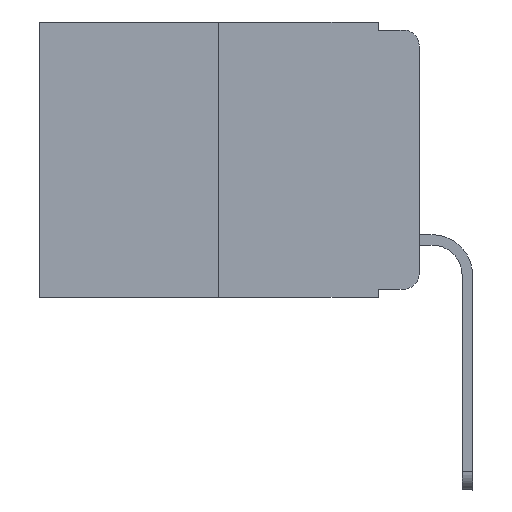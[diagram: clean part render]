
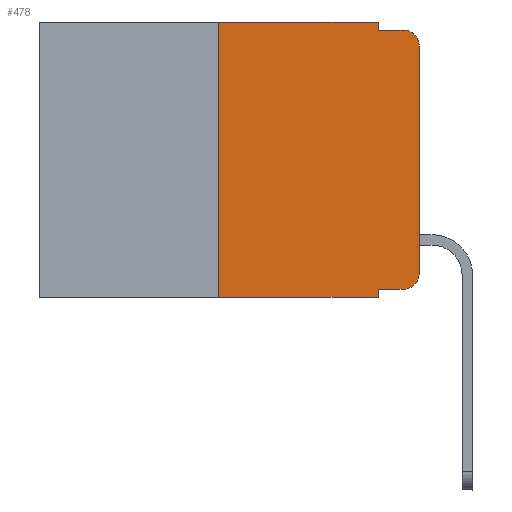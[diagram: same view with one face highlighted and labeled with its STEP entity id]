
A CAD part, left-side view. The second image highlights one B-rep face of the part: STEP entity #478.
In plain terms, the highlighted planar face has unit normal (-1, 0, 0).
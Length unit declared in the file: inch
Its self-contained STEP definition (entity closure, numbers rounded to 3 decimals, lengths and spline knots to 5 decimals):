
#27 = CARTESIAN_POINT ( 'NONE',  ( 0., 0.02, -0.03 ) ) ;
#33 = CARTESIAN_POINT ( 'NONE',  ( 0., 0.051, -0.01 ) ) ;
#117 = DIRECTION ( 'NONE',  ( -1., 0., 0. ) ) ;
#348 = DIRECTION ( 'NONE',  ( 0., 0., 1. ) ) ;
#376 = VERTEX_POINT ( 'NONE', #826 ) ;
#412 = CARTESIAN_POINT ( 'NONE',  ( 0., 0.051, 0. ) ) ;
#478 = ADVANCED_FACE ( 'NONE', ( #2706 ), #1529, .F. ) ;
#592 = ORIENTED_EDGE ( 'NONE', *, *, #7084, .F. ) ;
#634 = CARTESIAN_POINT ( 'NONE',  ( 0., 0., -0.313 ) ) ;
#696 = LINE ( 'NONE', #18897, #3251 ) ;
#716 = AXIS2_PLACEMENT_3D ( 'NONE', #27, #117, #4587 ) ;
#767 = DIRECTION ( 'NONE',  ( -1., 0., 0. ) ) ;
#826 = CARTESIAN_POINT ( 'NONE',  ( 0., 0., -0.03 ) ) ;
#844 = VERTEX_POINT ( 'NONE', #7108 ) ;
#1529 = PLANE ( 'NONE',  #13767 ) ;
#1797 = DIRECTION ( 'NONE',  ( 0., 0., -1. ) ) ;
#2015 = EDGE_CURVE ( 'NONE', #11160, #17276, #3012, .T. ) ;
#2037 = ORIENTED_EDGE ( 'NONE', *, *, #14180, .F. ) ;
#2569 = CIRCLE ( 'NONE', #716, 0.02 ) ;
#2580 = ORIENTED_EDGE ( 'NONE', *, *, #2015, .T. ) ;
#2706 = FACE_OUTER_BOUND ( 'NONE', #5067, .T. ) ;
#3012 = LINE ( 'NONE', #7434, #18607 ) ;
#3251 = VECTOR ( 'NONE', #11566, 39.37008 ) ;
#3405 = AXIS2_PLACEMENT_3D ( 'NONE', #15977, #767, #6865 ) ;
#4000 = EDGE_CURVE ( 'NONE', #11473, #17276, #696, .T. ) ;
#4437 = ORIENTED_EDGE ( 'NONE', *, *, #13019, .T. ) ;
#4450 = CARTESIAN_POINT ( 'NONE',  ( 0., 0., 0. ) ) ;
#4479 = EDGE_CURVE ( 'NONE', #18179, #11909, #17357, .T. ) ;
#4587 = DIRECTION ( 'NONE',  ( 0., 0., -1. ) ) ;
#5067 = EDGE_LOOP ( 'NONE', ( #4437, #7353, #2037, #13385, #9230, #592, #2580, #6376, #16366, #19621 ) ) ;
#5825 = EDGE_CURVE ( 'NONE', #376, #11939, #2569, .T. ) ;
#6079 = CARTESIAN_POINT ( 'NONE',  ( 0., 0.051, -0.333 ) ) ;
#6215 = CARTESIAN_POINT ( 'NONE',  ( 0., 0.473, 0. ) ) ;
#6376 = ORIENTED_EDGE ( 'NONE', *, *, #4000, .F. ) ;
#6865 = DIRECTION ( 'NONE',  ( 0., 0., -1. ) ) ;
#7060 = DIRECTION ( 'NONE',  ( 0., -1., 0. ) ) ;
#7084 = EDGE_CURVE ( 'NONE', #11160, #17067, #9528, .T. ) ;
#7108 = CARTESIAN_POINT ( 'NONE',  ( 0., 0.051, 0. ) ) ;
#7353 = ORIENTED_EDGE ( 'NONE', *, *, #5825, .T. ) ;
#7420 = CARTESIAN_POINT ( 'NONE',  ( 0., 0.473, 0. ) ) ;
#7434 = CARTESIAN_POINT ( 'NONE',  ( 0., 0.473, -0.343 ) ) ;
#7545 = CARTESIAN_POINT ( 'NONE',  ( 0., 0.25, -0.343 ) ) ;
#7975 = DIRECTION ( 'NONE',  ( 0., -1., 0. ) ) ;
#8148 = CARTESIAN_POINT ( 'NONE',  ( 0., 0.25, 0. ) ) ;
#8227 = VECTOR ( 'NONE', #7975, 39.37008 ) ;
#8346 = DIRECTION ( 'NONE',  ( 0., -1., 0. ) ) ;
#8631 = CARTESIAN_POINT ( 'NONE',  ( 0., 0.02, -0.333 ) ) ;
#8872 = VERTEX_POINT ( 'NONE', #33 ) ;
#8876 = VECTOR ( 'NONE', #15560, 39.37008 ) ;
#9021 = DIRECTION ( 'NONE',  ( 1., 0., 0. ) ) ;
#9230 = ORIENTED_EDGE ( 'NONE', *, *, #13568, .F. ) ;
#9360 = LINE ( 'NONE', #6079, #8227 ) ;
#9528 = LINE ( 'NONE', #18538, #8876 ) ;
#9903 = VECTOR ( 'NONE', #1797, 39.37008 ) ;
#10411 = LINE ( 'NONE', #7420, #15153 ) ;
#10870 = LINE ( 'NONE', #11333, #17044 ) ;
#11160 = VERTEX_POINT ( 'NONE', #7545 ) ;
#11333 = CARTESIAN_POINT ( 'NONE',  ( 0., 0.051, -0.01 ) ) ;
#11473 = VERTEX_POINT ( 'NONE', #17334 ) ;
#11566 = DIRECTION ( 'NONE',  ( 0., 0., -1. ) ) ;
#11721 = VECTOR ( 'NONE', #348, 39.37008 ) ;
#11909 = VERTEX_POINT ( 'NONE', #634 ) ;
#11939 = VERTEX_POINT ( 'NONE', #14442 ) ;
#12530 = EDGE_CURVE ( 'NONE', #11473, #18179, #9360, .T. ) ;
#13019 = EDGE_CURVE ( 'NONE', #11909, #376, #15078, .T. ) ;
#13385 = ORIENTED_EDGE ( 'NONE', *, *, #18861, .F. ) ;
#13568 = EDGE_CURVE ( 'NONE', #17067, #844, #10411, .T. ) ;
#13767 = AXIS2_PLACEMENT_3D ( 'NONE', #6215, #9021, #16438 ) ;
#14180 = EDGE_CURVE ( 'NONE', #8872, #11939, #10870, .T. ) ;
#14442 = CARTESIAN_POINT ( 'NONE',  ( 0., 0.02, -0.01 ) ) ;
#14547 = CARTESIAN_POINT ( 'NONE',  ( 0., 0.051, -0.343 ) ) ;
#15078 = LINE ( 'NONE', #4450, #11721 ) ;
#15153 = VECTOR ( 'NONE', #16528, 39.37008 ) ;
#15560 = DIRECTION ( 'NONE',  ( 0., 0., 1. ) ) ;
#15977 = CARTESIAN_POINT ( 'NONE',  ( 0., 0.02, -0.313 ) ) ;
#16366 = ORIENTED_EDGE ( 'NONE', *, *, #12530, .T. ) ;
#16438 = DIRECTION ( 'NONE',  ( 0., 0., -1. ) ) ;
#16528 = DIRECTION ( 'NONE',  ( 0., -1., 0. ) ) ;
#17044 = VECTOR ( 'NONE', #8346, 39.37008 ) ;
#17067 = VERTEX_POINT ( 'NONE', #8148 ) ;
#17276 = VERTEX_POINT ( 'NONE', #14547 ) ;
#17334 = CARTESIAN_POINT ( 'NONE',  ( 0., 0.051, -0.333 ) ) ;
#17357 = CIRCLE ( 'NONE', #3405, 0.02 ) ;
#18179 = VERTEX_POINT ( 'NONE', #8631 ) ;
#18510 = LINE ( 'NONE', #412, #9903 ) ;
#18538 = CARTESIAN_POINT ( 'NONE',  ( 0., 0.25, 0. ) ) ;
#18607 = VECTOR ( 'NONE', #7060, 39.37008 ) ;
#18861 = EDGE_CURVE ( 'NONE', #844, #8872, #18510, .T. ) ;
#18897 = CARTESIAN_POINT ( 'NONE',  ( 0., 0.051, 0. ) ) ;
#19621 = ORIENTED_EDGE ( 'NONE', *, *, #4479, .T. ) ;
